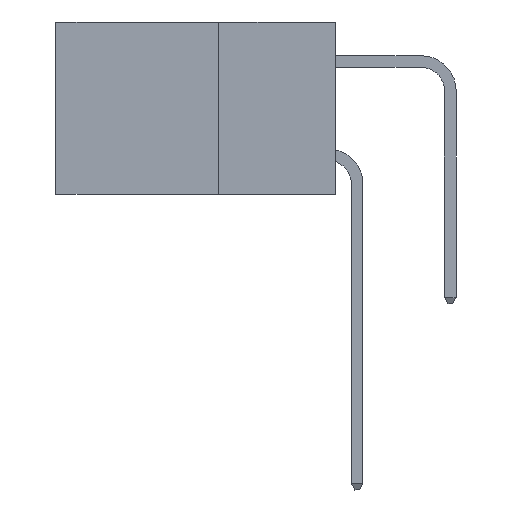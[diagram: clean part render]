
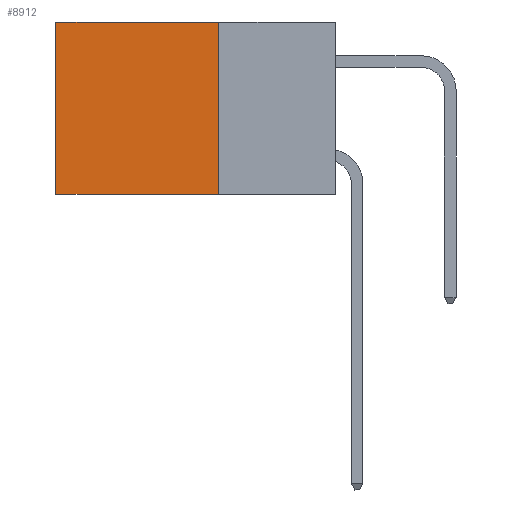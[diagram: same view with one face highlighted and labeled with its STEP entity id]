
A CAD part, left-side view. The second image highlights one B-rep face of the part: STEP entity #8912.
In plain terms, the highlighted planar face has unit normal (-1, 0, 0).
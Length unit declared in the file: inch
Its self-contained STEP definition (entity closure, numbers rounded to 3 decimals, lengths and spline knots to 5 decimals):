
#167 = CARTESIAN_POINT ( 'NONE',  ( 0.2875, 0.25, 0. ) ) ;
#605 = DIRECTION ( 'NONE',  ( 0., 1., 0. ) ) ;
#639 = CARTESIAN_POINT ( 'NONE',  ( 0.2875, 0.25, -0.37 ) ) ;
#837 = VECTOR ( 'NONE', #1028, 39.37008 ) ;
#937 = CARTESIAN_POINT ( 'NONE',  ( 0.2875, 0.25, 0. ) ) ;
#1028 = DIRECTION ( 'NONE',  ( 0., 1., 0. ) ) ;
#1519 = CARTESIAN_POINT ( 'NONE',  ( 0.2875, 0.6, -0.37 ) ) ;
#2084 = LINE ( 'NONE', #5694, #5178 ) ;
#2157 = DIRECTION ( 'NONE',  ( 1., 0., 0. ) ) ;
#2271 = VECTOR ( 'NONE', #4642, 39.37008 ) ;
#2898 = CARTESIAN_POINT ( 'NONE',  ( 0.2875, 0.6, 0. ) ) ;
#2987 = EDGE_CURVE ( 'NONE', #9383, #6307, #9330, .T. ) ;
#3005 = EDGE_CURVE ( 'NONE', #4193, #11348, #6043, .T. ) ;
#3047 = CARTESIAN_POINT ( 'NONE',  ( 0.2875, 0.25, -0.37 ) ) ;
#3129 = AXIS2_PLACEMENT_3D ( 'NONE', #12220, #2157, #9311 ) ;
#4193 = VERTEX_POINT ( 'NONE', #3047 ) ;
#4642 = DIRECTION ( 'NONE',  ( 0., 0., -1. ) ) ;
#4704 = ORIENTED_EDGE ( 'NONE', *, *, #2987, .T. ) ;
#4996 = ORIENTED_EDGE ( 'NONE', *, *, #3005, .F. ) ;
#5178 = VECTOR ( 'NONE', #11625, 39.37008 ) ;
#5556 = ORIENTED_EDGE ( 'NONE', *, *, #12388, .T. ) ;
#5694 = CARTESIAN_POINT ( 'NONE',  ( 0.2875, 0.6, 0. ) ) ;
#5706 = LINE ( 'NONE', #12635, #2271 ) ;
#6043 = LINE ( 'NONE', #639, #11302 ) ;
#6307 = VERTEX_POINT ( 'NONE', #2898 ) ;
#8311 = PLANE ( 'NONE',  #3129 ) ;
#8912 = ADVANCED_FACE ( 'NONE', ( #8922 ), #8311, .F. ) ;
#8922 = FACE_OUTER_BOUND ( 'NONE', #11336, .T. ) ;
#9114 = ORIENTED_EDGE ( 'NONE', *, *, #11354, .F. ) ;
#9311 = DIRECTION ( 'NONE',  ( 0., 0., -1. ) ) ;
#9330 = LINE ( 'NONE', #937, #837 ) ;
#9383 = VERTEX_POINT ( 'NONE', #167 ) ;
#11302 = VECTOR ( 'NONE', #605, 39.37008 ) ;
#11336 = EDGE_LOOP ( 'NONE', ( #5556, #4996, #9114, #4704 ) ) ;
#11348 = VERTEX_POINT ( 'NONE', #1519 ) ;
#11354 = EDGE_CURVE ( 'NONE', #9383, #4193, #5706, .T. ) ;
#11625 = DIRECTION ( 'NONE',  ( 0., 0., -1. ) ) ;
#12220 = CARTESIAN_POINT ( 'NONE',  ( 0.2875, 0.25, 0. ) ) ;
#12388 = EDGE_CURVE ( 'NONE', #6307, #11348, #2084, .T. ) ;
#12635 = CARTESIAN_POINT ( 'NONE',  ( 0.2875, 0.25, 0. ) ) ;
